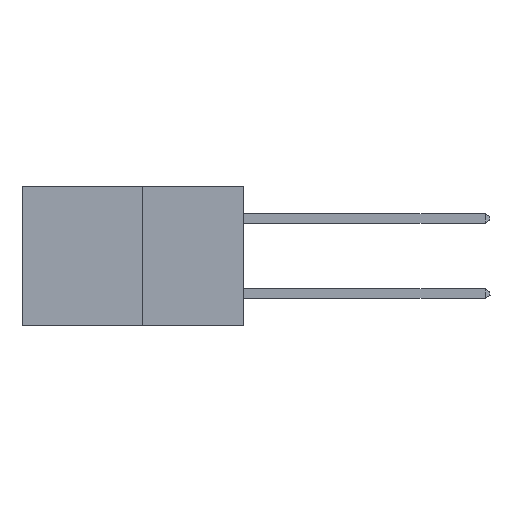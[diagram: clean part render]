
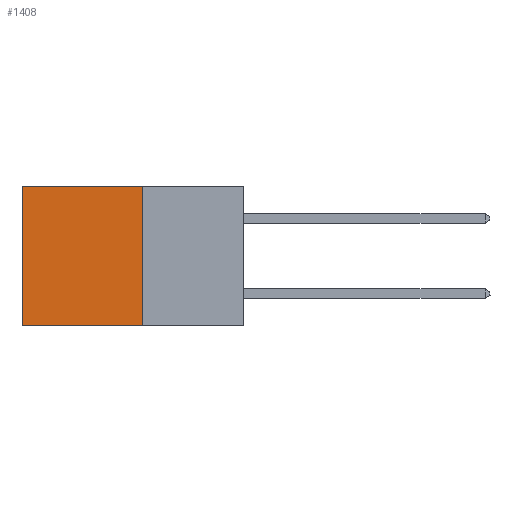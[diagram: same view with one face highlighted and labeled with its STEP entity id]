
A CAD part, left-side view. The second image highlights one B-rep face of the part: STEP entity #1408.
In plain terms, the highlighted planar face has unit normal (-1, 0, 0).
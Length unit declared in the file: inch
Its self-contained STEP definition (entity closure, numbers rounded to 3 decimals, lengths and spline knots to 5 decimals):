
#317 = PLANE ( 'NONE',  #7157 ) ;
#525 = CARTESIAN_POINT ( 'NONE',  ( 0.277, 0.59, -0.37 ) ) ;
#682 = VERTEX_POINT ( 'NONE', #525 ) ;
#812 = VERTEX_POINT ( 'NONE', #7868 ) ;
#868 = CARTESIAN_POINT ( 'NONE',  ( 0.277, 0.27, -0.37 ) ) ;
#1131 = CARTESIAN_POINT ( 'NONE',  ( 0.277, 0.59, 0. ) ) ;
#1230 = EDGE_CURVE ( 'NONE', #812, #682, #6323, .T. ) ;
#1408 = ADVANCED_FACE ( 'NONE', ( #2040 ), #317, .F. ) ;
#2040 = FACE_OUTER_BOUND ( 'NONE', #19135, .T. ) ;
#3961 = ORIENTED_EDGE ( 'NONE', *, *, #20622, .F. ) ;
#4740 = DIRECTION ( 'NONE',  ( 0., 1., 0. ) ) ;
#4938 = DIRECTION ( 'NONE',  ( 0., 0., -1. ) ) ;
#5323 = CARTESIAN_POINT ( 'NONE',  ( 0.277, 0.59, -0.37 ) ) ;
#6323 = LINE ( 'NONE', #11857, #23155 ) ;
#7157 = AXIS2_PLACEMENT_3D ( 'NONE', #868, #8448, #20715 ) ;
#7512 = ORIENTED_EDGE ( 'NONE', *, *, #9628, .T. ) ;
#7868 = CARTESIAN_POINT ( 'NONE',  ( 0.277, 0.27, -0.37 ) ) ;
#8448 = DIRECTION ( 'NONE',  ( 1., 0., 0. ) ) ;
#9628 = EDGE_CURVE ( 'NONE', #15049, #682, #26917, .T. ) ;
#9995 = EDGE_CURVE ( 'NONE', #13275, #15049, #23209, .T. ) ;
#11083 = CARTESIAN_POINT ( 'NONE',  ( 0.277, 0.27, -0.37 ) ) ;
#11857 = CARTESIAN_POINT ( 'NONE',  ( 0.277, 0.27, -0.37 ) ) ;
#11864 = LINE ( 'NONE', #11083, #17000 ) ;
#13113 = ORIENTED_EDGE ( 'NONE', *, *, #1230, .F. ) ;
#13275 = VERTEX_POINT ( 'NONE', #24213 ) ;
#14773 = VECTOR ( 'NONE', #4938, 39.37008 ) ;
#15049 = VERTEX_POINT ( 'NONE', #1131 ) ;
#17000 = VECTOR ( 'NONE', #28408, 39.37008 ) ;
#19135 = EDGE_LOOP ( 'NONE', ( #7512, #13113, #3961, #27972 ) ) ;
#20622 = EDGE_CURVE ( 'NONE', #13275, #812, #11864, .T. ) ;
#20715 = DIRECTION ( 'NONE',  ( 0., 0., -1. ) ) ;
#22425 = CARTESIAN_POINT ( 'NONE',  ( 0.277, 0.27, 0. ) ) ;
#22579 = VECTOR ( 'NONE', #4740, 39.37008 ) ;
#23155 = VECTOR ( 'NONE', #25270, 39.37008 ) ;
#23209 = LINE ( 'NONE', #22425, #22579 ) ;
#24213 = CARTESIAN_POINT ( 'NONE',  ( 0.277, 0.27, 0. ) ) ;
#25270 = DIRECTION ( 'NONE',  ( 0., 1., 0. ) ) ;
#26917 = LINE ( 'NONE', #5323, #14773 ) ;
#27972 = ORIENTED_EDGE ( 'NONE', *, *, #9995, .T. ) ;
#28408 = DIRECTION ( 'NONE',  ( 0., 0., -1. ) ) ;
